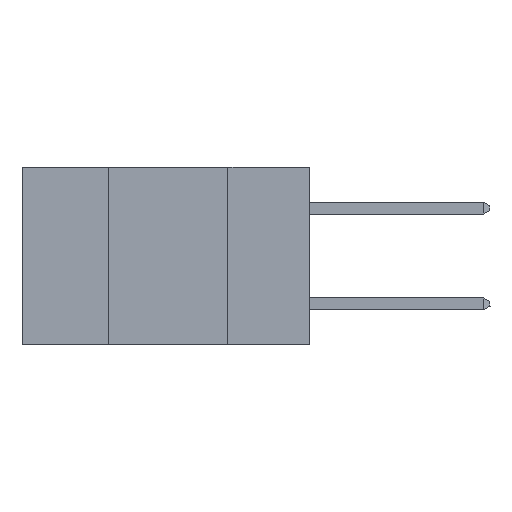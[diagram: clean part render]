
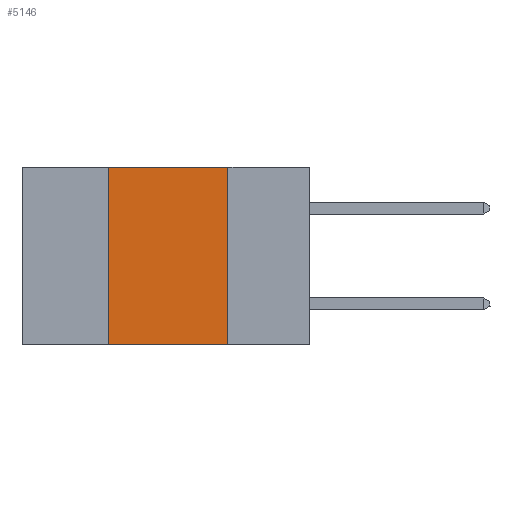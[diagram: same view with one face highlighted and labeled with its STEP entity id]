
A CAD part, left-side view. The second image highlights one B-rep face of the part: STEP entity #5146.
In plain terms, the highlighted planar face has unit normal (-1, 0, 0).
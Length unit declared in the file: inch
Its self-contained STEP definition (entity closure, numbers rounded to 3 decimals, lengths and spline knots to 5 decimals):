
#1500 = CARTESIAN_POINT ( 'NONE',  ( 0., 0.6, 0. ) ) ;
#4553 = DIRECTION ( 'NONE',  ( 0., 0., -1. ) ) ;
#4851 = ORIENTED_EDGE ( 'NONE', *, *, #37620, .F. ) ;
#4996 = DIRECTION ( 'NONE',  ( 0., -1., 0. ) ) ;
#5146 = ADVANCED_FACE ( 'NONE', ( #26956 ), #12298, .F. ) ;
#5665 = EDGE_CURVE ( 'NONE', #35762, #10203, #28033, .T. ) ;
#5778 = CARTESIAN_POINT ( 'NONE',  ( 0., 0.42, 0. ) ) ;
#7049 = DIRECTION ( 'NONE',  ( 1., 0., 0. ) ) ;
#7694 = ORIENTED_EDGE ( 'NONE', *, *, #5665, .F. ) ;
#7849 = AXIS2_PLACEMENT_3D ( 'NONE', #35835, #7049, #4553 ) ;
#8636 = ORIENTED_EDGE ( 'NONE', *, *, #28518, .T. ) ;
#10203 = VERTEX_POINT ( 'NONE', #5778 ) ;
#10617 = DIRECTION ( 'NONE',  ( 0., 0., -1. ) ) ;
#11150 = VERTEX_POINT ( 'NONE', #14523 ) ;
#12298 = PLANE ( 'NONE',  #7849 ) ;
#12902 = LINE ( 'NONE', #1500, #30564 ) ;
#13000 = CARTESIAN_POINT ( 'NONE',  ( 0., 0.42, 0. ) ) ;
#14029 = CARTESIAN_POINT ( 'NONE',  ( 0., 0.6, -0.37 ) ) ;
#14523 = CARTESIAN_POINT ( 'NONE',  ( 0., 0.17, 0. ) ) ;
#15724 = CARTESIAN_POINT ( 'NONE',  ( 0., 0.17, -0.37 ) ) ;
#16607 = LINE ( 'NONE', #28173, #20084 ) ;
#20084 = VECTOR ( 'NONE', #10617, 39.37008 ) ;
#21106 = CARTESIAN_POINT ( 'NONE',  ( 0., 0.42, -0.37 ) ) ;
#21614 = ORIENTED_EDGE ( 'NONE', *, *, #36515, .F. ) ;
#22447 = DIRECTION ( 'NONE',  ( 0., 0., 1. ) ) ;
#24495 = VERTEX_POINT ( 'NONE', #15724 ) ;
#25427 = DIRECTION ( 'NONE',  ( 0., -1., 0. ) ) ;
#26956 = FACE_OUTER_BOUND ( 'NONE', #31049, .T. ) ;
#28033 = LINE ( 'NONE', #13000, #32450 ) ;
#28173 = CARTESIAN_POINT ( 'NONE',  ( 0., 0.17, 0. ) ) ;
#28518 = EDGE_CURVE ( 'NONE', #35762, #24495, #34105, .T. ) ;
#29518 = VECTOR ( 'NONE', #25427, 39.37008 ) ;
#30564 = VECTOR ( 'NONE', #4996, 39.37008 ) ;
#31049 = EDGE_LOOP ( 'NONE', ( #21614, #4851, #7694, #8636 ) ) ;
#32450 = VECTOR ( 'NONE', #22447, 39.37008 ) ;
#34105 = LINE ( 'NONE', #14029, #29518 ) ;
#35762 = VERTEX_POINT ( 'NONE', #21106 ) ;
#35835 = CARTESIAN_POINT ( 'NONE',  ( 0., 0.6, 0. ) ) ;
#36515 = EDGE_CURVE ( 'NONE', #11150, #24495, #16607, .T. ) ;
#37620 = EDGE_CURVE ( 'NONE', #10203, #11150, #12902, .T. ) ;
